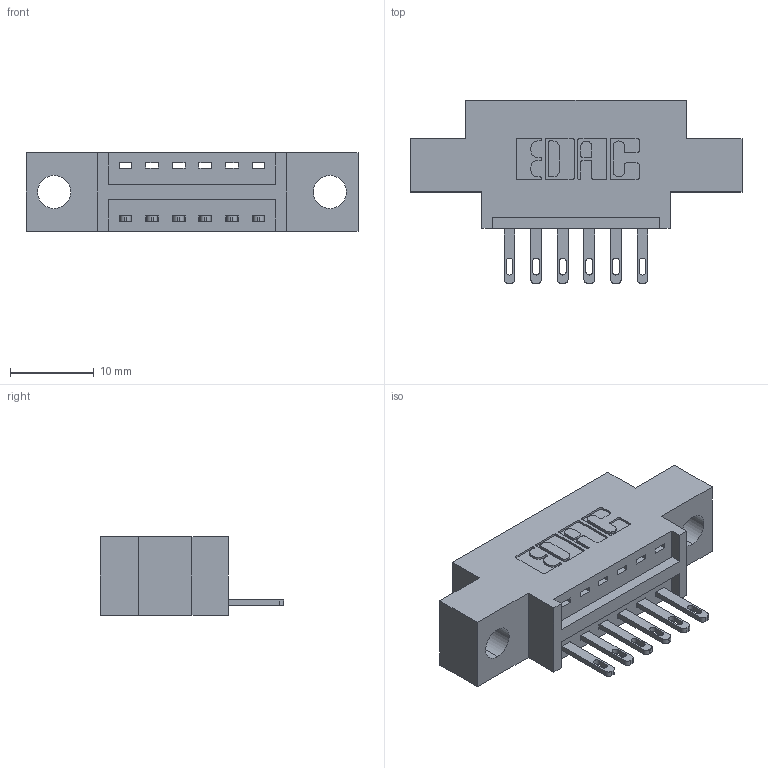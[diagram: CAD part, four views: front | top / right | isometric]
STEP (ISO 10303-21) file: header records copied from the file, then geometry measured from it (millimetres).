
FILE_DESCRIPTION (( 'STEP AP203' ), '1' );
FILE_NAME ('346-006-500-604.STEP', '2018-08-17T02:44:52', ( '' ), ( '' ), 'SwSTEP 2.0', 'SolidWorks 2016', '' );
FILE_SCHEMA (( 'CONFIG_CONTROL_DESIGN' ));
Length unit declared in the file: inch
Products named in the file (3): 346 Part_0.170 Offset - 0.156 Dia-TH; 345-292-001_345-293-100; 346-006-500-604
Assembly tree (7 placements, depth 2):
  346-006-500-604
    346 Part_0.170 Offset - 0.156 Dia-TH
    345-292-001_345-293-100  x6
Bounding box: 39.62 x 21.84 x 9.4 mm (x, y, z)
Volume: 3306.1 mm3; surface area: 3723 mm2
Topology: 7 solids, 7 shells, 450 faces, 1349 edges, 898 vertices
Faces by surface type: plane 284, cylinder 166
Entity records: 8635 total; most frequent: CARTESIAN_POINT 1498, ORIENTED_EDGE 1438, DIRECTION 1367, EDGE_CURVE 719, LINE 559, VECTOR 559, VERTEX_POINT 478, AXIS2_PLACEMENT_3D 404
